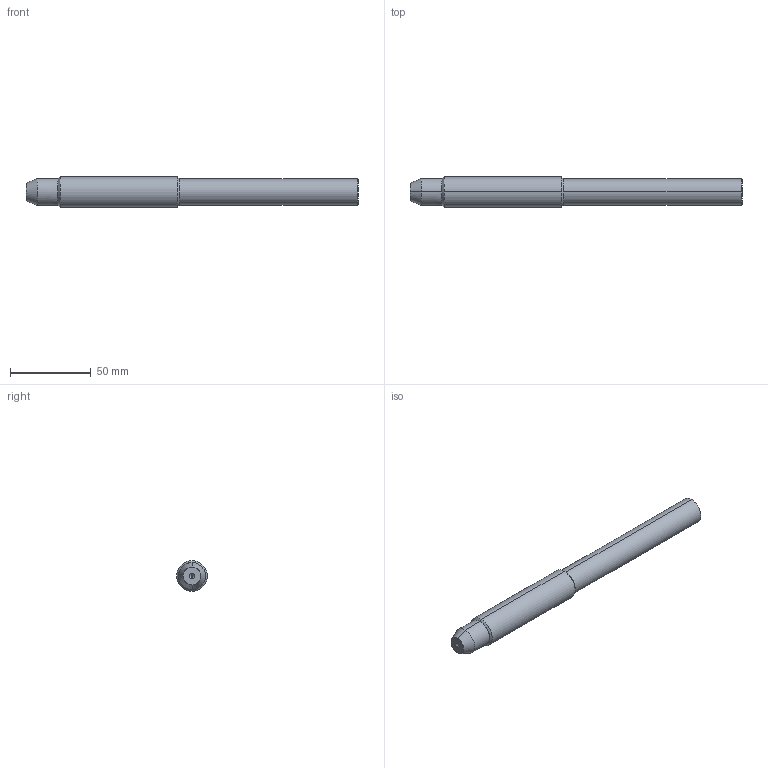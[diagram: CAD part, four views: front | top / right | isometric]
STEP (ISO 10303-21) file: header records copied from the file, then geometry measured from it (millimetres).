
FILE_DESCRIPTION (( 'STEP AP203' ), '1' );
FILE_NAME ('MOD9_V3_Top_Bolt.STEP', '2020-12-23T19:26:31', ( '' ), ( '' ), 'SwSTEP 2.0', 'SolidWorks 2019', '' );
FILE_SCHEMA (( 'CONFIG_CONTROL_DESIGN' ));
Length unit declared in the file: millimetre
Products named in the file (1): MOD9_V3_Top_Bolt
Bounding box: 206 x 19 x 19 mm (x, y, z)
Volume: 48255 mm3; surface area: 11518.5 mm2
Topology: 1 solids, 1 shells, 26 faces, 54 edges, 28 vertices
Faces by surface type: cone 12, bspline 6, cylinder 6, plane 2
Entity records: 1034 total; most frequent: CARTESIAN_POINT 444, DIRECTION 112, ORIENTED_EDGE 100, EDGE_CURVE 50, AXIS2_PLACEMENT_3D 47, EDGE_LOOP 28, VERTEX_POINT 28, ADVANCED_FACE 26
